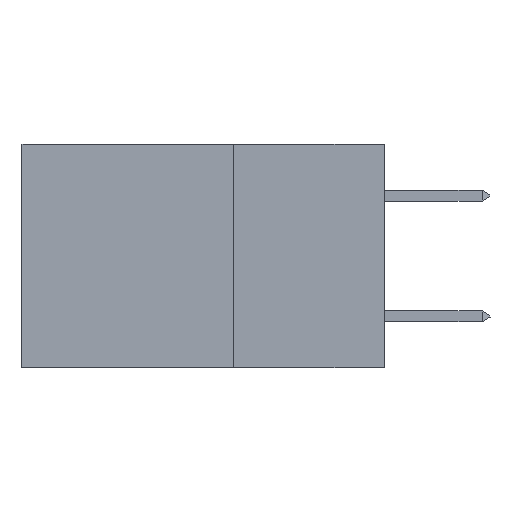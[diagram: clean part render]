
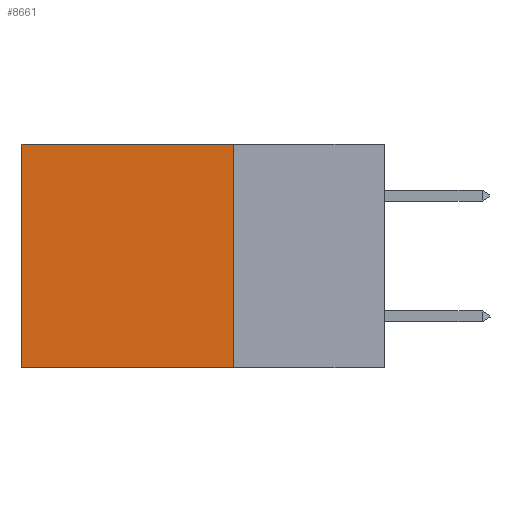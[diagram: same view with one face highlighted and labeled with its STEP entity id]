
A CAD part, left-side view. The second image highlights one B-rep face of the part: STEP entity #8661.
In plain terms, the highlighted planar face has unit normal (-1, 0, 0).
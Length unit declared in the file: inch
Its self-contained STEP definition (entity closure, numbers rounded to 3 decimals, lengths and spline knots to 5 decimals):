
#188 = CARTESIAN_POINT ( 'NONE',  ( 0.2875, 0.25, 0. ) ) ;
#722 = DIRECTION ( 'NONE',  ( 0., 0., -1. ) ) ;
#873 = LINE ( 'NONE', #188, #3883 ) ;
#1425 = LINE ( 'NONE', #9861, #16238 ) ;
#1535 = EDGE_CURVE ( 'NONE', #20303, #20584, #1425, .T. ) ;
#3883 = VECTOR ( 'NONE', #19201, 39.37008 ) ;
#4131 = CARTESIAN_POINT ( 'NONE',  ( 0.2875, 0.6, 0. ) ) ;
#5193 = EDGE_CURVE ( 'NONE', #7072, #20303, #5963, .T. ) ;
#5963 = LINE ( 'NONE', #14890, #15244 ) ;
#6891 = LINE ( 'NONE', #9620, #17308 ) ;
#7072 = VERTEX_POINT ( 'NONE', #10970 ) ;
#8661 = ADVANCED_FACE ( 'NONE', ( #17539 ), #15239, .F. ) ;
#9620 = CARTESIAN_POINT ( 'NONE',  ( 0.2875, 0.6, 0. ) ) ;
#9861 = CARTESIAN_POINT ( 'NONE',  ( 0.2875, 0.25, -0.37 ) ) ;
#9873 = CARTESIAN_POINT ( 'NONE',  ( 0.2875, 0.6, -0.37 ) ) ;
#10015 = DIRECTION ( 'NONE',  ( 0., 1., 0. ) ) ;
#10029 = VERTEX_POINT ( 'NONE', #4131 ) ;
#10970 = CARTESIAN_POINT ( 'NONE',  ( 0.2875, 0.25, 0. ) ) ;
#11284 = ORIENTED_EDGE ( 'NONE', *, *, #15958, .T. ) ;
#13284 = DIRECTION ( 'NONE',  ( 0., 0., -1. ) ) ;
#14851 = CARTESIAN_POINT ( 'NONE',  ( 0.2875, 0.25, -0.37 ) ) ;
#14890 = CARTESIAN_POINT ( 'NONE',  ( 0.2875, 0.25, 0. ) ) ;
#15239 = PLANE ( 'NONE',  #21495 ) ;
#15244 = VECTOR ( 'NONE', #13284, 39.37008 ) ;
#15958 = EDGE_CURVE ( 'NONE', #10029, #20584, #6891, .T. ) ;
#16238 = VECTOR ( 'NONE', #10015, 39.37008 ) ;
#17255 = DIRECTION ( 'NONE',  ( 1., 0., 0. ) ) ;
#17308 = VECTOR ( 'NONE', #722, 39.37008 ) ;
#17427 = ORIENTED_EDGE ( 'NONE', *, *, #19557, .T. ) ;
#17539 = FACE_OUTER_BOUND ( 'NONE', #21761, .T. ) ;
#19201 = DIRECTION ( 'NONE',  ( 0., 1., 0. ) ) ;
#19557 = EDGE_CURVE ( 'NONE', #7072, #10029, #873, .T. ) ;
#20303 = VERTEX_POINT ( 'NONE', #14851 ) ;
#20584 = VERTEX_POINT ( 'NONE', #9873 ) ;
#20616 = CARTESIAN_POINT ( 'NONE',  ( 0.2875, 0.25, 0. ) ) ;
#20699 = ORIENTED_EDGE ( 'NONE', *, *, #5193, .F. ) ;
#21495 = AXIS2_PLACEMENT_3D ( 'NONE', #20616, #17255, #22222 ) ;
#21530 = ORIENTED_EDGE ( 'NONE', *, *, #1535, .F. ) ;
#21761 = EDGE_LOOP ( 'NONE', ( #11284, #21530, #20699, #17427 ) ) ;
#22222 = DIRECTION ( 'NONE',  ( 0., 0., -1. ) ) ;
